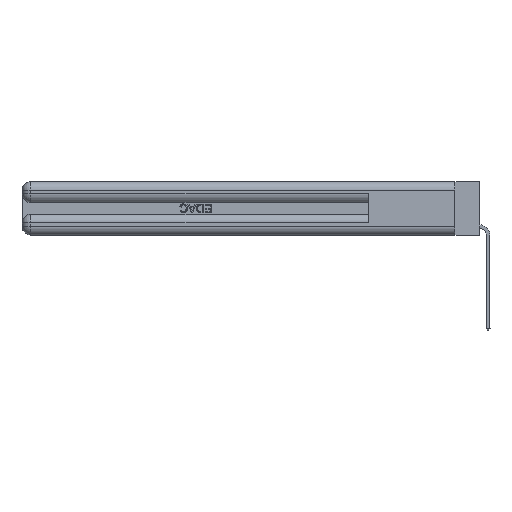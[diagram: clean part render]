
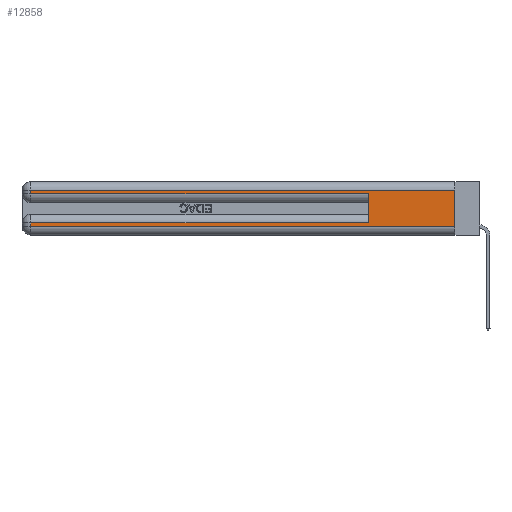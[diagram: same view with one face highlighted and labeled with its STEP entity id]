
A CAD part, left-side view. The second image highlights one B-rep face of the part: STEP entity #12858.
In plain terms, the highlighted planar face has unit normal (-1, 0, 0).
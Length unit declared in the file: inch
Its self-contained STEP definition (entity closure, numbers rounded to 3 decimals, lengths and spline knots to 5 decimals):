
#145 = CARTESIAN_POINT ( 'NONE',  ( 0., 0., 0.37 ) ) ;
#290 = ORIENTED_EDGE ( 'NONE', *, *, #12556, .T. ) ;
#308 = VECTOR ( 'NONE', #8393, 39.37008 ) ;
#608 = VERTEX_POINT ( 'NONE', #16266 ) ;
#826 = VERTEX_POINT ( 'NONE', #8820 ) ;
#1612 = CARTESIAN_POINT ( 'NONE',  ( 0., 2.94, 0.31 ) ) ;
#2377 = EDGE_CURVE ( 'NONE', #7842, #608, #25960, .T. ) ;
#3412 = CARTESIAN_POINT ( 'NONE',  ( 0., 2.94, 0.285 ) ) ;
#3868 = ORIENTED_EDGE ( 'NONE', *, *, #5541, .T. ) ;
#4816 = VECTOR ( 'NONE', #14493, 39.37008 ) ;
#5541 = EDGE_CURVE ( 'NONE', #23957, #8714, #11668, .T. ) ;
#5948 = CARTESIAN_POINT ( 'NONE',  ( 0., 0., 0.37 ) ) ;
#6311 = VERTEX_POINT ( 'NONE', #9702 ) ;
#6326 = CARTESIAN_POINT ( 'NONE',  ( 0., 0., 0.085 ) ) ;
#6883 = VECTOR ( 'NONE', #26089, 39.37008 ) ;
#7016 = LINE ( 'NONE', #6326, #308 ) ;
#7713 = CARTESIAN_POINT ( 'NONE',  ( 0., 0.6, 0.145 ) ) ;
#7842 = VERTEX_POINT ( 'NONE', #14588 ) ;
#8004 = DIRECTION ( 'NONE',  ( 1., 0., 0. ) ) ;
#8106 = ORIENTED_EDGE ( 'NONE', *, *, #19497, .F. ) ;
#8393 = DIRECTION ( 'NONE',  ( 0., 1., 0. ) ) ;
#8465 = CARTESIAN_POINT ( 'NONE',  ( 0., 0., 0.285 ) ) ;
#8505 = EDGE_LOOP ( 'NONE', ( #19491, #290, #21129, #3868, #8106, #12086, #19709, #19823 ) ) ;
#8714 = VERTEX_POINT ( 'NONE', #15874 ) ;
#8820 = CARTESIAN_POINT ( 'NONE',  ( 0., 0., 0.06 ) ) ;
#9014 = DIRECTION ( 'NONE',  ( 0., 1., 0. ) ) ;
#9702 = CARTESIAN_POINT ( 'NONE',  ( 0., 0.6, 0.085 ) ) ;
#11668 = LINE ( 'NONE', #8465, #21917 ) ;
#12086 = ORIENTED_EDGE ( 'NONE', *, *, #12322, .T. ) ;
#12322 = EDGE_CURVE ( 'NONE', #6311, #7842, #7016, .T. ) ;
#12556 = EDGE_CURVE ( 'NONE', #20927, #13825, #16308, .T. ) ;
#12858 = ADVANCED_FACE ( 'NONE', ( #18881 ), #18230, .F. ) ;
#13160 = CARTESIAN_POINT ( 'NONE',  ( 0., 0., 0.31 ) ) ;
#13754 = CARTESIAN_POINT ( 'NONE',  ( 0., 2.94, 0.37 ) ) ;
#13825 = VERTEX_POINT ( 'NONE', #1612 ) ;
#13956 = DIRECTION ( 'NONE',  ( 0., 0., -1. ) ) ;
#14493 = DIRECTION ( 'NONE',  ( 0., 0., -1. ) ) ;
#14588 = CARTESIAN_POINT ( 'NONE',  ( 0., 2.94, 0.085 ) ) ;
#15874 = CARTESIAN_POINT ( 'NONE',  ( 0., 0.6, 0.285 ) ) ;
#16266 = CARTESIAN_POINT ( 'NONE',  ( 0., 2.94, 0.06 ) ) ;
#16308 = LINE ( 'NONE', #13160, #21773 ) ;
#17925 = CARTESIAN_POINT ( 'NONE',  ( 0., 0., 0.31 ) ) ;
#18230 = PLANE ( 'NONE',  #23797 ) ;
#18710 = DIRECTION ( 'NONE',  ( 0., -1., 0. ) ) ;
#18881 = FACE_OUTER_BOUND ( 'NONE', #8505, .T. ) ;
#19491 = ORIENTED_EDGE ( 'NONE', *, *, #22105, .F. ) ;
#19497 = EDGE_CURVE ( 'NONE', #6311, #8714, #19579, .T. ) ;
#19579 = LINE ( 'NONE', #7713, #24415 ) ;
#19709 = ORIENTED_EDGE ( 'NONE', *, *, #2377, .T. ) ;
#19823 = ORIENTED_EDGE ( 'NONE', *, *, #20428, .T. ) ;
#19840 = VECTOR ( 'NONE', #26542, 39.37008 ) ;
#20428 = EDGE_CURVE ( 'NONE', #608, #826, #25329, .T. ) ;
#20927 = VERTEX_POINT ( 'NONE', #17925 ) ;
#21129 = ORIENTED_EDGE ( 'NONE', *, *, #25149, .T. ) ;
#21773 = VECTOR ( 'NONE', #9014, 39.37008 ) ;
#21917 = VECTOR ( 'NONE', #18710, 39.37008 ) ;
#22105 = EDGE_CURVE ( 'NONE', #20927, #826, #26042, .T. ) ;
#22357 = DIRECTION ( 'NONE',  ( 0., 0., -1. ) ) ;
#22629 = LINE ( 'NONE', #13754, #6883 ) ;
#23797 = AXIS2_PLACEMENT_3D ( 'NONE', #5948, #8004, #22357 ) ;
#23957 = VERTEX_POINT ( 'NONE', #3412 ) ;
#24184 = DIRECTION ( 'NONE',  ( 0., 0., 1. ) ) ;
#24415 = VECTOR ( 'NONE', #24184, 39.37008 ) ;
#25149 = EDGE_CURVE ( 'NONE', #13825, #23957, #22629, .T. ) ;
#25329 = LINE ( 'NONE', #26632, #19840 ) ;
#25960 = LINE ( 'NONE', #26281, #26598 ) ;
#26042 = LINE ( 'NONE', #145, #4816 ) ;
#26089 = DIRECTION ( 'NONE',  ( 0., 0., -1. ) ) ;
#26281 = CARTESIAN_POINT ( 'NONE',  ( 0., 2.94, 0.37 ) ) ;
#26542 = DIRECTION ( 'NONE',  ( 0., -1., 0. ) ) ;
#26598 = VECTOR ( 'NONE', #13956, 39.37008 ) ;
#26632 = CARTESIAN_POINT ( 'NONE',  ( 0., 0., 0.06 ) ) ;
